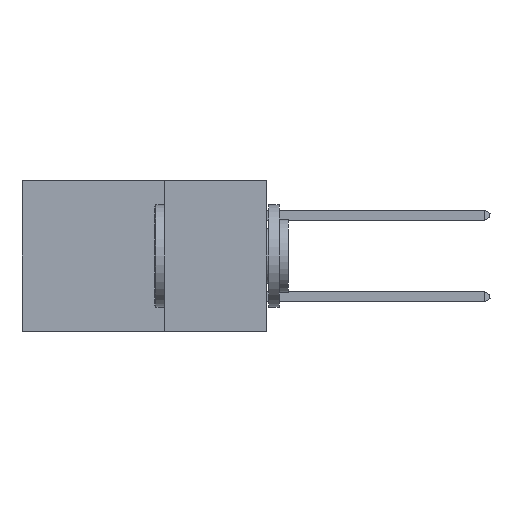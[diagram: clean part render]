
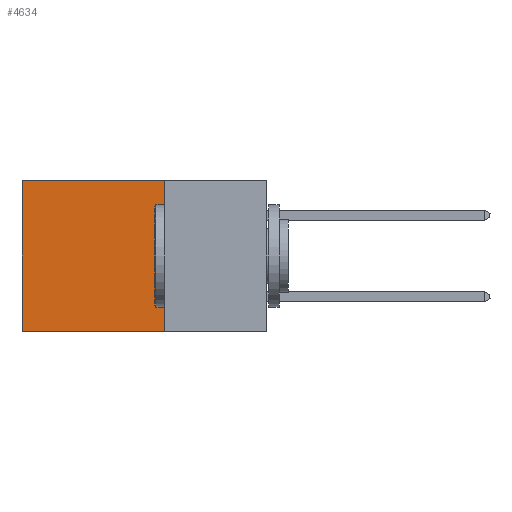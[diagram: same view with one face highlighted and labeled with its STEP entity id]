
A CAD part, left-side view. The second image highlights one B-rep face of the part: STEP entity #4634.
In plain terms, the highlighted planar face has unit normal (-1, 0, 0).
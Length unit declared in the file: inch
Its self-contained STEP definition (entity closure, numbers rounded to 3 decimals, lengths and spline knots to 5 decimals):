
#54 = EDGE_CURVE ( 'NONE', #26624, #7183, #12158, .T. ) ;
#1096 = LINE ( 'NONE', #24205, #24994 ) ;
#1987 = DIRECTION ( 'NONE',  ( 0., 0., -1. ) ) ;
#2045 = DIRECTION ( 'NONE',  ( 1., 0., 0. ) ) ;
#2843 = ORIENTED_EDGE ( 'NONE', *, *, #14639, .T. ) ;
#4634 = ADVANCED_FACE ( 'NONE', ( #20386 ), #13295, .F. ) ;
#5844 = CARTESIAN_POINT ( 'NONE',  ( 0.2875, 0.6, 0. ) ) ;
#5998 = CARTESIAN_POINT ( 'NONE',  ( 0.2875, 0.6, -0.37 ) ) ;
#6242 = CARTESIAN_POINT ( 'NONE',  ( 0.2875, 0.25, 0. ) ) ;
#6432 = VECTOR ( 'NONE', #10134, 39.37008 ) ;
#6903 = EDGE_CURVE ( 'NONE', #12493, #26624, #1096, .T. ) ;
#7183 = VERTEX_POINT ( 'NONE', #5998 ) ;
#8643 = LINE ( 'NONE', #27128, #10333 ) ;
#8945 = LINE ( 'NONE', #6242, #25745 ) ;
#10134 = DIRECTION ( 'NONE',  ( 0., 1., 0. ) ) ;
#10333 = VECTOR ( 'NONE', #12316, 39.37008 ) ;
#11721 = ORIENTED_EDGE ( 'NONE', *, *, #6903, .F. ) ;
#12158 = LINE ( 'NONE', #14171, #6432 ) ;
#12271 = ORIENTED_EDGE ( 'NONE', *, *, #23279, .T. ) ;
#12316 = DIRECTION ( 'NONE',  ( 0., 0., -1. ) ) ;
#12493 = VERTEX_POINT ( 'NONE', #19316 ) ;
#13295 = PLANE ( 'NONE',  #13372 ) ;
#13372 = AXIS2_PLACEMENT_3D ( 'NONE', #26767, #2045, #1987 ) ;
#14171 = CARTESIAN_POINT ( 'NONE',  ( 0.2875, 0.25, -0.37 ) ) ;
#14517 = VERTEX_POINT ( 'NONE', #5844 ) ;
#14639 = EDGE_CURVE ( 'NONE', #14517, #7183, #8643, .T. ) ;
#17202 = ORIENTED_EDGE ( 'NONE', *, *, #54, .F. ) ;
#19316 = CARTESIAN_POINT ( 'NONE',  ( 0.2875, 0.25, 0. ) ) ;
#19387 = DIRECTION ( 'NONE',  ( 0., 1., 0. ) ) ;
#19892 = DIRECTION ( 'NONE',  ( 0., 0., -1. ) ) ;
#20386 = FACE_OUTER_BOUND ( 'NONE', #21280, .T. ) ;
#21280 = EDGE_LOOP ( 'NONE', ( #2843, #17202, #11721, #12271 ) ) ;
#23279 = EDGE_CURVE ( 'NONE', #12493, #14517, #8945, .T. ) ;
#24205 = CARTESIAN_POINT ( 'NONE',  ( 0.2875, 0.25, 0. ) ) ;
#24994 = VECTOR ( 'NONE', #19892, 39.37008 ) ;
#25745 = VECTOR ( 'NONE', #19387, 39.37008 ) ;
#26624 = VERTEX_POINT ( 'NONE', #26952 ) ;
#26767 = CARTESIAN_POINT ( 'NONE',  ( 0.2875, 0.25, 0. ) ) ;
#26952 = CARTESIAN_POINT ( 'NONE',  ( 0.2875, 0.25, -0.37 ) ) ;
#27128 = CARTESIAN_POINT ( 'NONE',  ( 0.2875, 0.6, 0. ) ) ;
